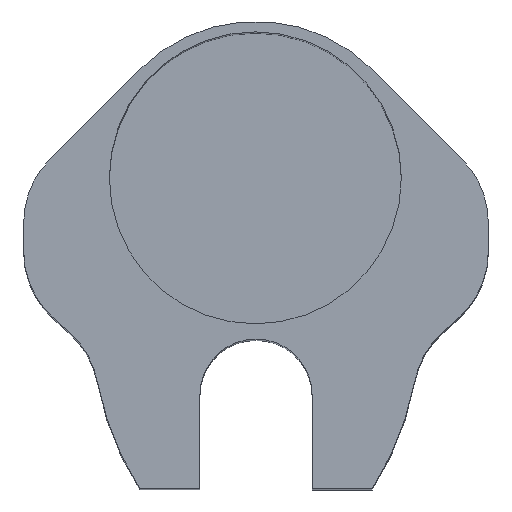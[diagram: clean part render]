
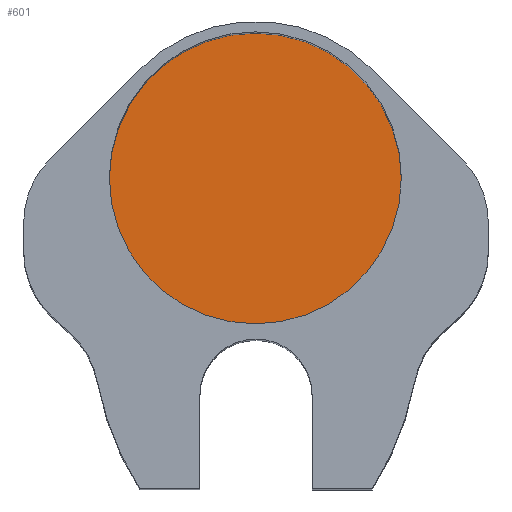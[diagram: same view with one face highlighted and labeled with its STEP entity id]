
A CAD part, top view. The second image highlights one B-rep face of the part: STEP entity #601.
In plain terms, the highlighted planar face has unit normal (0, 0, 1).
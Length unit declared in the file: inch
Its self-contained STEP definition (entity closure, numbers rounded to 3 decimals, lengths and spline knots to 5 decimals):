
#7 = ORIENTED_EDGE ( 'NONE', *, *, #359, .F. ) ;
#44 = CIRCLE ( 'NONE', #457, 0.65 ) ;
#66 = CARTESIAN_POINT ( 'NONE',  ( 5.62271, 7.60667, 2.0401 ) ) ;
#137 = ORIENTED_EDGE ( 'NONE', *, *, #1035, .F. ) ;
#169 = CARTESIAN_POINT ( 'NONE',  ( 4.32271, 7.60667, 2.0401 ) ) ;
#264 = CARTESIAN_POINT ( 'NONE',  ( 4.97271, 7.60667, 2.0401 ) ) ;
#359 = EDGE_CURVE ( 'NONE', #756, #721, #44, .T. ) ;
#435 = DIRECTION ( 'NONE',  ( 1., 0., 0. ) ) ;
#457 = AXIS2_PLACEMENT_3D ( 'NONE', #994, #1015, #716 ) ;
#477 = CIRCLE ( 'NONE', #533, 0.65 ) ;
#533 = AXIS2_PLACEMENT_3D ( 'NONE', #590, #598, #577 ) ;
#577 = DIRECTION ( 'NONE',  ( 1., 0., 0. ) ) ;
#590 = CARTESIAN_POINT ( 'NONE',  ( 4.97271, 7.60667, 2.0401 ) ) ;
#598 = DIRECTION ( 'NONE',  ( 0., 0., -1. ) ) ;
#601 = ADVANCED_FACE ( 'NONE', ( #613 ), #1022, .F. ) ;
#613 = FACE_OUTER_BOUND ( 'NONE', #705, .T. ) ;
#666 = DIRECTION ( 'NONE',  ( 0., 0., -1. ) ) ;
#705 = EDGE_LOOP ( 'NONE', ( #7, #137 ) ) ;
#716 = DIRECTION ( 'NONE',  ( 1., 0., 0. ) ) ;
#721 = VERTEX_POINT ( 'NONE', #169 ) ;
#756 = VERTEX_POINT ( 'NONE', #66 ) ;
#774 = AXIS2_PLACEMENT_3D ( 'NONE', #264, #666, #435 ) ;
#994 = CARTESIAN_POINT ( 'NONE',  ( 4.97271, 7.60667, 2.0401 ) ) ;
#1015 = DIRECTION ( 'NONE',  ( 0., 0., -1. ) ) ;
#1022 = PLANE ( 'NONE',  #774 ) ;
#1035 = EDGE_CURVE ( 'NONE', #721, #756, #477, .T. ) ;
